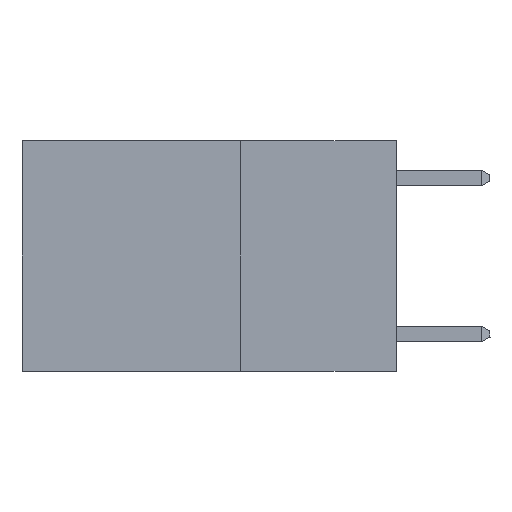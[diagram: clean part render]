
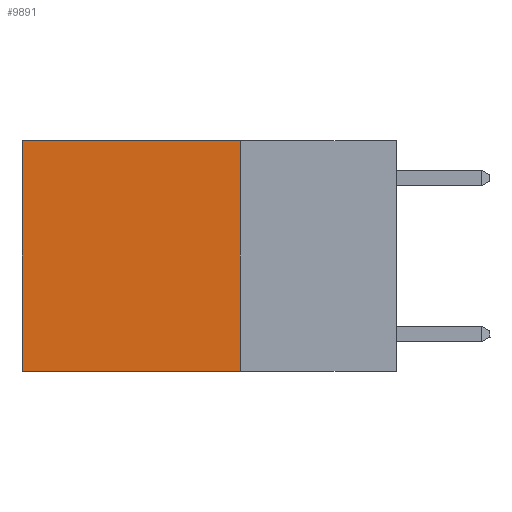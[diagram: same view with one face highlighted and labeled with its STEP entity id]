
A CAD part, left-side view. The second image highlights one B-rep face of the part: STEP entity #9891.
In plain terms, the highlighted planar face has unit normal (-1, 0, 0).
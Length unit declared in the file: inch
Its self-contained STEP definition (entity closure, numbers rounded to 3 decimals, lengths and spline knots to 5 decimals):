
#1424 = VECTOR ( 'NONE', #8532, 39.37008 ) ;
#1923 = VECTOR ( 'NONE', #5391, 39.37008 ) ;
#2275 = CARTESIAN_POINT ( 'NONE',  ( 0.2625, 0.25, -0.37 ) ) ;
#2843 = CARTESIAN_POINT ( 'NONE',  ( 0.2625, 0.6, 0. ) ) ;
#3067 = CARTESIAN_POINT ( 'NONE',  ( 0.2625, 0.25, 0. ) ) ;
#4634 = EDGE_CURVE ( 'NONE', #25615, #26232, #7823, .T. ) ;
#5391 = DIRECTION ( 'NONE',  ( 0., 0., -1. ) ) ;
#5509 = ORIENTED_EDGE ( 'NONE', *, *, #4634, .T. ) ;
#5697 = VERTEX_POINT ( 'NONE', #2275 ) ;
#6773 = EDGE_CURVE ( 'NONE', #25615, #5697, #26980, .T. ) ;
#7566 = CARTESIAN_POINT ( 'NONE',  ( 0.2625, 0.6, 0. ) ) ;
#7823 = LINE ( 'NONE', #10723, #1424 ) ;
#8532 = DIRECTION ( 'NONE',  ( 0., 1., 0. ) ) ;
#9564 = LINE ( 'NONE', #26458, #25440 ) ;
#9891 = ADVANCED_FACE ( 'NONE', ( #12667 ), #25242, .F. ) ;
#10723 = CARTESIAN_POINT ( 'NONE',  ( 0.2625, 0.25, 0. ) ) ;
#11581 = ORIENTED_EDGE ( 'NONE', *, *, #16223, .F. ) ;
#12045 = LINE ( 'NONE', #7566, #1923 ) ;
#12315 = DIRECTION ( 'NONE',  ( 1., 0., 0. ) ) ;
#12667 = FACE_OUTER_BOUND ( 'NONE', #19235, .T. ) ;
#12925 = ORIENTED_EDGE ( 'NONE', *, *, #6773, .F. ) ;
#13832 = ORIENTED_EDGE ( 'NONE', *, *, #24325, .T. ) ;
#14201 = CARTESIAN_POINT ( 'NONE',  ( 0.2625, 0.25, 0. ) ) ;
#16223 = EDGE_CURVE ( 'NONE', #5697, #18717, #9564, .T. ) ;
#16596 = AXIS2_PLACEMENT_3D ( 'NONE', #25149, #12315, #27403 ) ;
#18426 = CARTESIAN_POINT ( 'NONE',  ( 0.2625, 0.6, -0.37 ) ) ;
#18717 = VERTEX_POINT ( 'NONE', #18426 ) ;
#19235 = EDGE_LOOP ( 'NONE', ( #13832, #11581, #12925, #5509 ) ) ;
#24300 = DIRECTION ( 'NONE',  ( 0., 1., 0. ) ) ;
#24325 = EDGE_CURVE ( 'NONE', #26232, #18717, #12045, .T. ) ;
#25149 = CARTESIAN_POINT ( 'NONE',  ( 0.2625, 0.25, 0. ) ) ;
#25242 = PLANE ( 'NONE',  #16596 ) ;
#25440 = VECTOR ( 'NONE', #24300, 39.37008 ) ;
#25615 = VERTEX_POINT ( 'NONE', #3067 ) ;
#26232 = VERTEX_POINT ( 'NONE', #2843 ) ;
#26289 = VECTOR ( 'NONE', #27236, 39.37008 ) ;
#26458 = CARTESIAN_POINT ( 'NONE',  ( 0.2625, 0.25, -0.37 ) ) ;
#26980 = LINE ( 'NONE', #14201, #26289 ) ;
#27236 = DIRECTION ( 'NONE',  ( 0., 0., -1. ) ) ;
#27403 = DIRECTION ( 'NONE',  ( 0., 0., -1. ) ) ;
